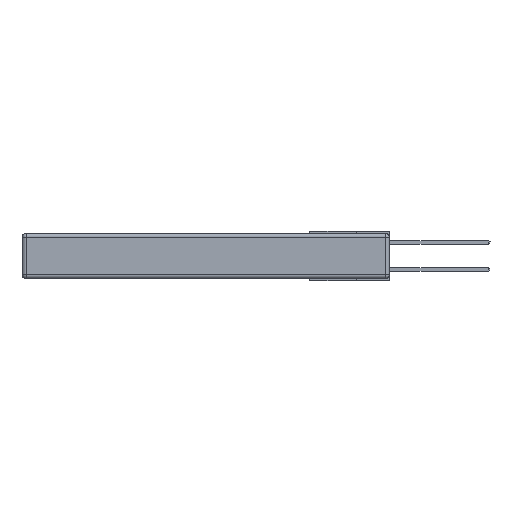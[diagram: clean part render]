
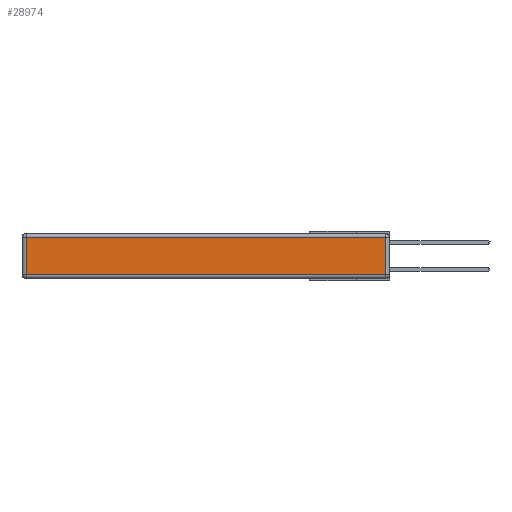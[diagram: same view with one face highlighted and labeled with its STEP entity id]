
A CAD part, left-side view. The second image highlights one B-rep face of the part: STEP entity #28974.
In plain terms, the highlighted planar face has unit normal (-1, 0, 0).
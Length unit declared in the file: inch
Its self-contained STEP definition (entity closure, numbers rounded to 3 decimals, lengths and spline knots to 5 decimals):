
#2773 = DIRECTION ( 'NONE',  ( 0., 0., 1. ) ) ;
#5387 = VECTOR ( 'NONE', #13469, 39.37008 ) ;
#7666 = LINE ( 'NONE', #18146, #5387 ) ;
#8243 = CARTESIAN_POINT ( 'NONE',  ( 0., 2.72, -0.03 ) ) ;
#8419 = FACE_OUTER_BOUND ( 'NONE', #15662, .T. ) ;
#8477 = CARTESIAN_POINT ( 'NONE',  ( 0., 0.03, -0.343 ) ) ;
#8923 = PLANE ( 'NONE',  #21532 ) ;
#9891 = VERTEX_POINT ( 'NONE', #23667 ) ;
#10453 = DIRECTION ( 'NONE',  ( 0., -1., 0. ) ) ;
#10477 = DIRECTION ( 'NONE',  ( 0., 1., 0. ) ) ;
#12527 = VECTOR ( 'NONE', #10477, 39.37008 ) ;
#12766 = ORIENTED_EDGE ( 'NONE', *, *, #20049, .T. ) ;
#13469 = DIRECTION ( 'NONE',  ( 0., 0., -1. ) ) ;
#14439 = DIRECTION ( 'NONE',  ( 0., 0., 1. ) ) ;
#14716 = ORIENTED_EDGE ( 'NONE', *, *, #15198, .T. ) ;
#15198 = EDGE_CURVE ( 'NONE', #9891, #15276, #18237, .T. ) ;
#15276 = VERTEX_POINT ( 'NONE', #8243 ) ;
#15662 = EDGE_LOOP ( 'NONE', ( #24887, #30260, #14716, #12766 ) ) ;
#16827 = VERTEX_POINT ( 'NONE', #29035 ) ;
#17833 = EDGE_CURVE ( 'NONE', #19996, #9891, #28382, .T. ) ;
#18146 = CARTESIAN_POINT ( 'NONE',  ( 0., 2.72, -0.343 ) ) ;
#18237 = LINE ( 'NONE', #25073, #12527 ) ;
#18498 = EDGE_CURVE ( 'NONE', #16827, #19996, #22634, .T. ) ;
#19996 = VERTEX_POINT ( 'NONE', #25115 ) ;
#20049 = EDGE_CURVE ( 'NONE', #15276, #16827, #7666, .T. ) ;
#21532 = AXIS2_PLACEMENT_3D ( 'NONE', #30812, #24390, #2773 ) ;
#22634 = LINE ( 'NONE', #25159, #28708 ) ;
#23667 = CARTESIAN_POINT ( 'NONE',  ( 0., 0.03, -0.03 ) ) ;
#24390 = DIRECTION ( 'NONE',  ( -1., 0., 0. ) ) ;
#24887 = ORIENTED_EDGE ( 'NONE', *, *, #18498, .T. ) ;
#25073 = CARTESIAN_POINT ( 'NONE',  ( 0., 2.75, -0.03 ) ) ;
#25115 = CARTESIAN_POINT ( 'NONE',  ( 0., 0.03, -0.313 ) ) ;
#25159 = CARTESIAN_POINT ( 'NONE',  ( 0., 0., -0.313 ) ) ;
#26112 = VECTOR ( 'NONE', #14439, 39.37008 ) ;
#28382 = LINE ( 'NONE', #8477, #26112 ) ;
#28708 = VECTOR ( 'NONE', #10453, 39.37008 ) ;
#28974 = ADVANCED_FACE ( 'NONE', ( #8419 ), #8923, .T. ) ;
#29035 = CARTESIAN_POINT ( 'NONE',  ( 0., 2.72, -0.313 ) ) ;
#30260 = ORIENTED_EDGE ( 'NONE', *, *, #17833, .T. ) ;
#30812 = CARTESIAN_POINT ( 'NONE',  ( 0., 0., -0.343 ) ) ;
